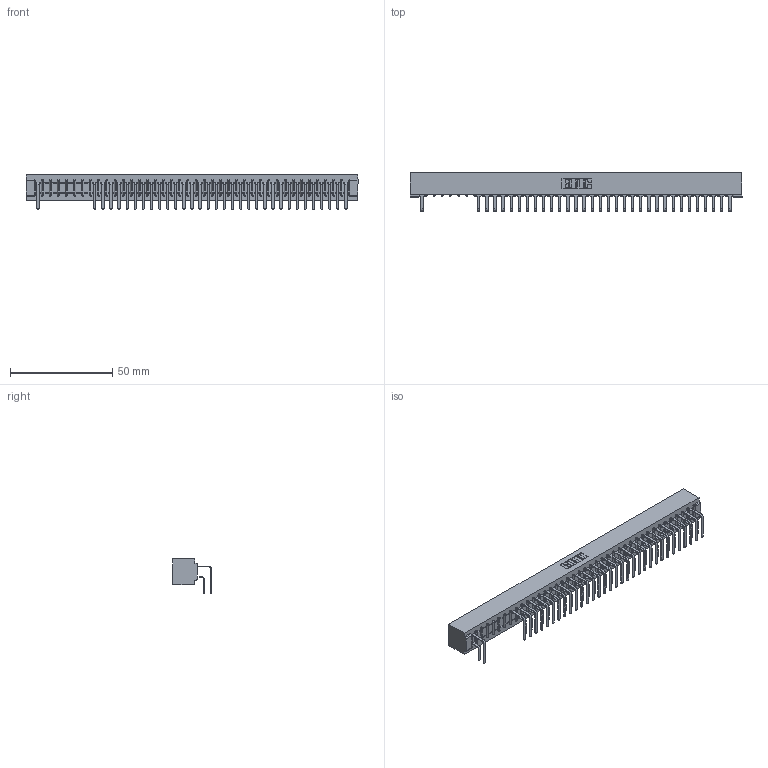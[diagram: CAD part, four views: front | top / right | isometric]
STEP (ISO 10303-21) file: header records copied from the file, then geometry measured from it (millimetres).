
FILE_DESCRIPTION (( 'STEP AP203' ), '1' );
FILE_NAME ('307-078-558-201.STEP', '2018-08-06T17:58:52', ( '' ), ( '' ), 'SwSTEP 2.0', 'SolidWorks 2016', '' );
FILE_SCHEMA (( 'CONFIG_CONTROL_DESIGN' ));
Length unit declared in the file: inch
Products named in the file (4): 307-290-001_558 - 2 (Single); 307-078-558-201; 307 Part_No Mounting Lugs; 307-290-001_558 559 - 1 (Single)
Assembly tree (66 placements, depth 2):
  307-078-558-201
    307 Part_No Mounting Lugs
    307-290-001_558 559 - 1 (Single)  x32
    307-290-001_558 - 2 (Single)  x33
Bounding box: 162.41 x 18.96 x 16.8 mm (x, y, z)
Volume: 17917.9 mm3; surface area: 22762.2 mm2
Topology: 66 solids, 66 shells, 3530 faces, 9945 edges, 6434 vertices
Faces by surface type: plane 2289, cylinder 1161, sphere 80
Entity records: 35805 total; most frequent: CARTESIAN_POINT 5912, ORIENTED_EDGE 5870, DIRECTION 5777, EDGE_CURVE 2935, VECTOR 2251, LINE 2251, VERTEX_POINT 1898, AXIS2_PLACEMENT_3D 1763
